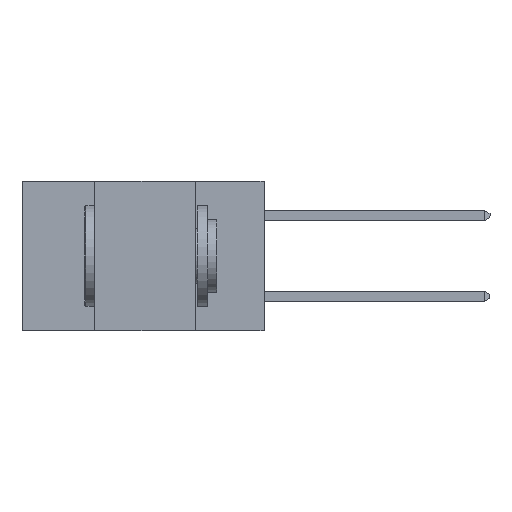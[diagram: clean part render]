
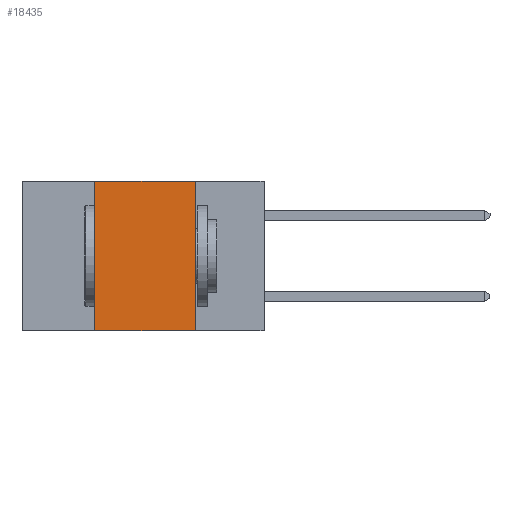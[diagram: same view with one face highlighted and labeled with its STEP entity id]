
A CAD part, left-side view. The second image highlights one B-rep face of the part: STEP entity #18435.
In plain terms, the highlighted planar face has unit normal (-1, 0, 0).
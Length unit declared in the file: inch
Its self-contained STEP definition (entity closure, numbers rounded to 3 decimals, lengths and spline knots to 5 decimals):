
#411 = VERTEX_POINT ( 'NONE', #14203 ) ;
#1700 = VERTEX_POINT ( 'NONE', #2691 ) ;
#1712 = EDGE_LOOP ( 'NONE', ( #10196, #9524, #5489, #22960 ) ) ;
#1718 = CARTESIAN_POINT ( 'NONE',  ( 0., 0.6, 0. ) ) ;
#1772 = VECTOR ( 'NONE', #27351, 39.37008 ) ;
#2691 = CARTESIAN_POINT ( 'NONE',  ( 0., 0.42, 0. ) ) ;
#2882 = DIRECTION ( 'NONE',  ( 0., 0., -1. ) ) ;
#3116 = VECTOR ( 'NONE', #11497, 39.37008 ) ;
#3370 = LINE ( 'NONE', #11509, #25844 ) ;
#4009 = AXIS2_PLACEMENT_3D ( 'NONE', #26120, #9193, #24394 ) ;
#5489 = ORIENTED_EDGE ( 'NONE', *, *, #27124, .F. ) ;
#8655 = CARTESIAN_POINT ( 'NONE',  ( 0., 0.17, -0.37 ) ) ;
#9193 = DIRECTION ( 'NONE',  ( 1., 0., 0. ) ) ;
#9300 = CARTESIAN_POINT ( 'NONE',  ( 0., 0.6, -0.37 ) ) ;
#9524 = ORIENTED_EDGE ( 'NONE', *, *, #22391, .F. ) ;
#10196 = ORIENTED_EDGE ( 'NONE', *, *, #17956, .F. ) ;
#10420 = CARTESIAN_POINT ( 'NONE',  ( 0., 0.42, -0.37 ) ) ;
#11497 = DIRECTION ( 'NONE',  ( 0., -1., 0. ) ) ;
#11509 = CARTESIAN_POINT ( 'NONE',  ( 0., 0.17, 0. ) ) ;
#13413 = LINE ( 'NONE', #16380, #1772 ) ;
#14203 = CARTESIAN_POINT ( 'NONE',  ( 0., 0.17, 0. ) ) ;
#14388 = VERTEX_POINT ( 'NONE', #10420 ) ;
#15327 = VECTOR ( 'NONE', #19018, 39.37008 ) ;
#16380 = CARTESIAN_POINT ( 'NONE',  ( 0., 0.42, 0. ) ) ;
#17811 = PLANE ( 'NONE',  #4009 ) ;
#17956 = EDGE_CURVE ( 'NONE', #411, #22804, #3370, .T. ) ;
#18435 = ADVANCED_FACE ( 'NONE', ( #25825 ), #17811, .F. ) ;
#19018 = DIRECTION ( 'NONE',  ( 0., -1., 0. ) ) ;
#19092 = LINE ( 'NONE', #9300, #3116 ) ;
#20401 = LINE ( 'NONE', #1718, #15327 ) ;
#22003 = EDGE_CURVE ( 'NONE', #14388, #22804, #19092, .T. ) ;
#22391 = EDGE_CURVE ( 'NONE', #1700, #411, #20401, .T. ) ;
#22804 = VERTEX_POINT ( 'NONE', #8655 ) ;
#22960 = ORIENTED_EDGE ( 'NONE', *, *, #22003, .T. ) ;
#24394 = DIRECTION ( 'NONE',  ( 0., 0., -1. ) ) ;
#25825 = FACE_OUTER_BOUND ( 'NONE', #1712, .T. ) ;
#25844 = VECTOR ( 'NONE', #2882, 39.37008 ) ;
#26120 = CARTESIAN_POINT ( 'NONE',  ( 0., 0.6, 0. ) ) ;
#27124 = EDGE_CURVE ( 'NONE', #14388, #1700, #13413, .T. ) ;
#27351 = DIRECTION ( 'NONE',  ( 0., 0., 1. ) ) ;
